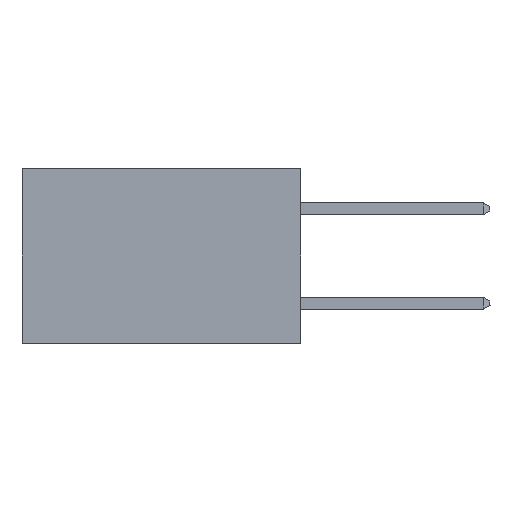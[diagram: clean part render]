
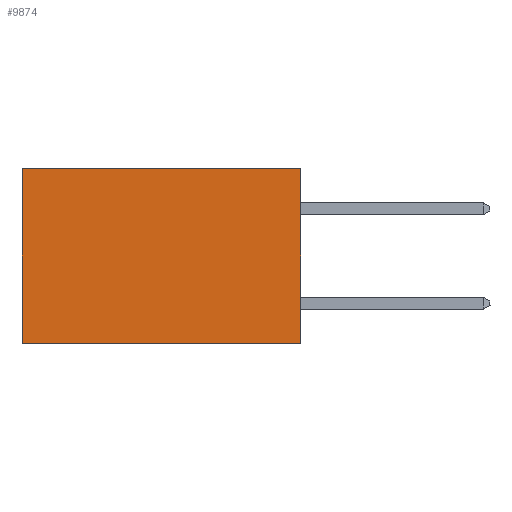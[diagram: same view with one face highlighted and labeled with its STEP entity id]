
A CAD part, left-side view. The second image highlights one B-rep face of the part: STEP entity #9874.
In plain terms, the highlighted planar face has unit normal (-1, 0, 0).
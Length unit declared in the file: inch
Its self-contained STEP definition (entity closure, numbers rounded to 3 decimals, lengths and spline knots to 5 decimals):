
#365 = CARTESIAN_POINT ( 'NONE',  ( 0.277, 0., -0.37 ) ) ;
#1030 = EDGE_CURVE ( 'NONE', #12124, #11347, #12309, .T. ) ;
#1110 = CARTESIAN_POINT ( 'NONE',  ( 0.277, 0.59, 0. ) ) ;
#1354 = AXIS2_PLACEMENT_3D ( 'NONE', #14821, #9067, #2267 ) ;
#2267 = DIRECTION ( 'NONE',  ( 0., 0., -1. ) ) ;
#2659 = LINE ( 'NONE', #9646, #5309 ) ;
#3259 = FACE_OUTER_BOUND ( 'NONE', #5903, .T. ) ;
#3995 = EDGE_CURVE ( 'NONE', #11858, #4692, #12021, .T. ) ;
#4692 = VERTEX_POINT ( 'NONE', #13711 ) ;
#4816 = VECTOR ( 'NONE', #13787, 39.37008 ) ;
#4928 = DIRECTION ( 'NONE',  ( 0., 1., 0. ) ) ;
#5309 = VECTOR ( 'NONE', #10803, 39.37008 ) ;
#5903 = EDGE_LOOP ( 'NONE', ( #9957, #11317, #10413, #11873 ) ) ;
#5939 = EDGE_CURVE ( 'NONE', #11347, #4692, #8241, .T. ) ;
#6329 = VECTOR ( 'NONE', #10716, 39.37008 ) ;
#7921 = PLANE ( 'NONE',  #1354 ) ;
#8241 = LINE ( 'NONE', #11743, #10173 ) ;
#9067 = DIRECTION ( 'NONE',  ( 1., 0., 0. ) ) ;
#9520 = CARTESIAN_POINT ( 'NONE',  ( 0.277, 0.59, -0.37 ) ) ;
#9646 = CARTESIAN_POINT ( 'NONE',  ( 0.277, 0., 0. ) ) ;
#9874 = ADVANCED_FACE ( 'NONE', ( #3259 ), #7921, .F. ) ;
#9957 = ORIENTED_EDGE ( 'NONE', *, *, #3995, .T. ) ;
#10173 = VECTOR ( 'NONE', #4928, 39.37008 ) ;
#10413 = ORIENTED_EDGE ( 'NONE', *, *, #1030, .F. ) ;
#10679 = CARTESIAN_POINT ( 'NONE',  ( 0.277, 0., 0. ) ) ;
#10716 = DIRECTION ( 'NONE',  ( 0., 0., -1. ) ) ;
#10803 = DIRECTION ( 'NONE',  ( 0., 1., 0. ) ) ;
#10892 = CARTESIAN_POINT ( 'NONE',  ( 0.277, 0., -0.37 ) ) ;
#11317 = ORIENTED_EDGE ( 'NONE', *, *, #5939, .F. ) ;
#11347 = VERTEX_POINT ( 'NONE', #365 ) ;
#11467 = EDGE_CURVE ( 'NONE', #12124, #11858, #2659, .T. ) ;
#11743 = CARTESIAN_POINT ( 'NONE',  ( 0.277, 0., -0.37 ) ) ;
#11858 = VERTEX_POINT ( 'NONE', #1110 ) ;
#11873 = ORIENTED_EDGE ( 'NONE', *, *, #11467, .T. ) ;
#12021 = LINE ( 'NONE', #9520, #6329 ) ;
#12124 = VERTEX_POINT ( 'NONE', #10679 ) ;
#12309 = LINE ( 'NONE', #10892, #4816 ) ;
#13711 = CARTESIAN_POINT ( 'NONE',  ( 0.277, 0.59, -0.37 ) ) ;
#13787 = DIRECTION ( 'NONE',  ( 0., 0., -1. ) ) ;
#14821 = CARTESIAN_POINT ( 'NONE',  ( 0.277, 0., -0.37 ) ) ;
